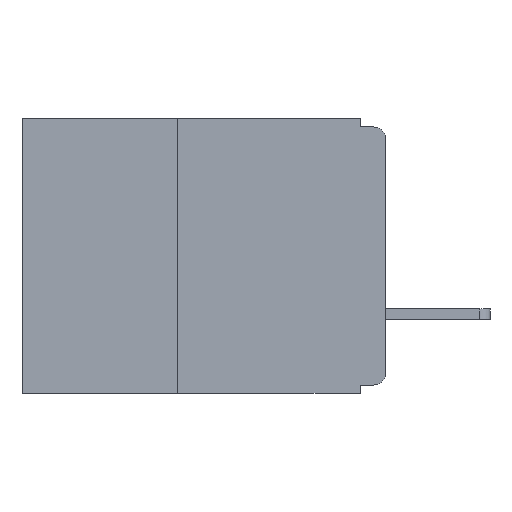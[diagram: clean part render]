
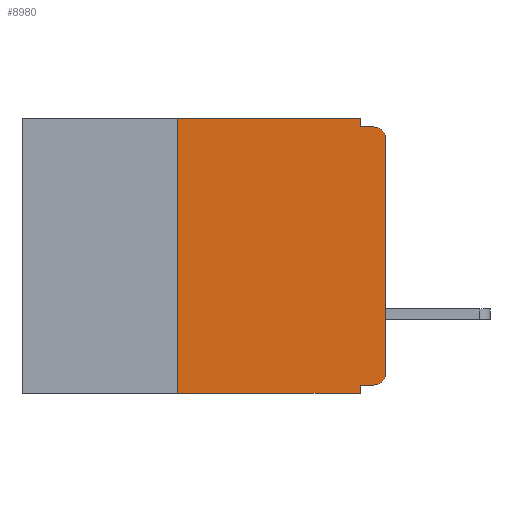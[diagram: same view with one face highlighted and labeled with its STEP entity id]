
A CAD part, left-side view. The second image highlights one B-rep face of the part: STEP entity #8980.
In plain terms, the highlighted planar face has unit normal (-1, 0, 0).
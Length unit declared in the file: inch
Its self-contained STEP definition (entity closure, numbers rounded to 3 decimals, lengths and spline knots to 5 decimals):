
#140 = CARTESIAN_POINT ( 'NONE',  ( 0., 0.031, -0.01 ) ) ;
#210 = AXIS2_PLACEMENT_3D ( 'NONE', #26010, #25913, #25876 ) ;
#274 = EDGE_CURVE ( 'NONE', #29803, #27475, #3256, .T. ) ;
#433 = ORIENTED_EDGE ( 'NONE', *, *, #26208, .T. ) ;
#924 = CARTESIAN_POINT ( 'NONE',  ( 0., 0.031, -0.33 ) ) ;
#1409 = VERTEX_POINT ( 'NONE', #28042 ) ;
#1490 = VECTOR ( 'NONE', #11071, 39.37008 ) ;
#3256 = LINE ( 'NONE', #18717, #8362 ) ;
#3645 = DIRECTION ( 'NONE',  ( 0., 0., 1. ) ) ;
#4241 = VECTOR ( 'NONE', #13066, 39.37008 ) ;
#4512 = LINE ( 'NONE', #16980, #16951 ) ;
#4658 = EDGE_CURVE ( 'NONE', #27873, #8387, #24845, .T. ) ;
#5413 = VERTEX_POINT ( 'NONE', #924 ) ;
#5503 = EDGE_LOOP ( 'NONE', ( #16473, #433, #24006, #29252, #25175, #14495, #21458, #30095, #6450, #28640 ) ) ;
#5930 = CARTESIAN_POINT ( 'NONE',  ( 0., 0.437, -0.33 ) ) ;
#6450 = ORIENTED_EDGE ( 'NONE', *, *, #13812, .F. ) ;
#6608 = CARTESIAN_POINT ( 'NONE',  ( 0., 0.015, -0.01 ) ) ;
#8142 = CARTESIAN_POINT ( 'NONE',  ( 0., 0.015, -0.025 ) ) ;
#8357 = VECTOR ( 'NONE', #3645, 39.37008 ) ;
#8362 = VECTOR ( 'NONE', #19721, 39.37008 ) ;
#8387 = VERTEX_POINT ( 'NONE', #30942 ) ;
#8980 = ADVANCED_FACE ( 'NONE', ( #16807 ), #26097, .F. ) ;
#9494 = CARTESIAN_POINT ( 'NONE',  ( 0., 0.015, -0.305 ) ) ;
#9584 = VECTOR ( 'NONE', #22092, 39.37008 ) ;
#9661 = CARTESIAN_POINT ( 'NONE',  ( 0., 0.031, -0.32 ) ) ;
#10629 = DIRECTION ( 'NONE',  ( 0., 0., -1. ) ) ;
#10862 = LINE ( 'NONE', #30079, #4241 ) ;
#11071 = DIRECTION ( 'NONE',  ( 0., 0., -1. ) ) ;
#11941 = DIRECTION ( 'NONE',  ( 0., 0., -1. ) ) ;
#13066 = DIRECTION ( 'NONE',  ( 0., -1., 0. ) ) ;
#13812 = EDGE_CURVE ( 'NONE', #22123, #22270, #4512, .T. ) ;
#13885 = EDGE_CURVE ( 'NONE', #16780, #29803, #15384, .T. ) ;
#14495 = ORIENTED_EDGE ( 'NONE', *, *, #27711, .F. ) ;
#15384 = LINE ( 'NONE', #26950, #9584 ) ;
#15468 = LINE ( 'NONE', #15939, #1490 ) ;
#15740 = CIRCLE ( 'NONE', #26552, 0.015 ) ;
#15939 = CARTESIAN_POINT ( 'NONE',  ( 0., 0.031, -0.33 ) ) ;
#16473 = ORIENTED_EDGE ( 'NONE', *, *, #4658, .T. ) ;
#16761 = VERTEX_POINT ( 'NONE', #6608 ) ;
#16780 = VERTEX_POINT ( 'NONE', #23722 ) ;
#16807 = FACE_OUTER_BOUND ( 'NONE', #5503, .T. ) ;
#16812 = CARTESIAN_POINT ( 'NONE',  ( 0., 0., -0.305 ) ) ;
#16951 = VECTOR ( 'NONE', #19457, 39.37008 ) ;
#16980 = CARTESIAN_POINT ( 'NONE',  ( 0., 0., -0.32 ) ) ;
#17456 = VECTOR ( 'NONE', #18286, 39.37008 ) ;
#18286 = DIRECTION ( 'NONE',  ( 0., -1., 0. ) ) ;
#18717 = CARTESIAN_POINT ( 'NONE',  ( 0., 0.031, 0. ) ) ;
#18892 = CARTESIAN_POINT ( 'NONE',  ( 0., 0.015, -0.32 ) ) ;
#19457 = DIRECTION ( 'NONE',  ( 0., 1., 0. ) ) ;
#19721 = DIRECTION ( 'NONE',  ( 0., 0., -1. ) ) ;
#20587 = CARTESIAN_POINT ( 'NONE',  ( 0., 0.031, 0. ) ) ;
#20899 = CARTESIAN_POINT ( 'NONE',  ( 0., 0.25, -0.33 ) ) ;
#21458 = ORIENTED_EDGE ( 'NONE', *, *, #25149, .T. ) ;
#22092 = DIRECTION ( 'NONE',  ( 0., -1., 0. ) ) ;
#22123 = VERTEX_POINT ( 'NONE', #18892 ) ;
#22270 = VERTEX_POINT ( 'NONE', #9661 ) ;
#23187 = CARTESIAN_POINT ( 'NONE',  ( 0., 0., 0. ) ) ;
#23360 = DIRECTION ( 'NONE',  ( 0., 0., 1. ) ) ;
#23722 = CARTESIAN_POINT ( 'NONE',  ( 0., 0.25, 0. ) ) ;
#24006 = ORIENTED_EDGE ( 'NONE', *, *, #25105, .F. ) ;
#24845 = LINE ( 'NONE', #23187, #30454 ) ;
#25105 = EDGE_CURVE ( 'NONE', #27475, #16761, #10862, .T. ) ;
#25149 = EDGE_CURVE ( 'NONE', #1409, #5413, #28792, .T. ) ;
#25175 = ORIENTED_EDGE ( 'NONE', *, *, #13885, .F. ) ;
#25314 = DIRECTION ( 'NONE',  ( -1., 0., 0. ) ) ;
#25789 = EDGE_CURVE ( 'NONE', #22270, #5413, #15468, .T. ) ;
#25876 = DIRECTION ( 'NONE',  ( 0., 0., -1. ) ) ;
#25913 = DIRECTION ( 'NONE',  ( 1., 0., 0. ) ) ;
#26010 = CARTESIAN_POINT ( 'NONE',  ( 0., 0.437, 0. ) ) ;
#26097 = PLANE ( 'NONE',  #210 ) ;
#26208 = EDGE_CURVE ( 'NONE', #8387, #16761, #27601, .T. ) ;
#26552 = AXIS2_PLACEMENT_3D ( 'NONE', #9494, #26610, #11941 ) ;
#26610 = DIRECTION ( 'NONE',  ( -1., 0., 0. ) ) ;
#26950 = CARTESIAN_POINT ( 'NONE',  ( 0., 0.437, 0. ) ) ;
#27314 = EDGE_CURVE ( 'NONE', #22123, #27873, #15740, .T. ) ;
#27323 = AXIS2_PLACEMENT_3D ( 'NONE', #8142, #25314, #10629 ) ;
#27475 = VERTEX_POINT ( 'NONE', #140 ) ;
#27601 = CIRCLE ( 'NONE', #27323, 0.015 ) ;
#27711 = EDGE_CURVE ( 'NONE', #1409, #16780, #27867, .T. ) ;
#27867 = LINE ( 'NONE', #20899, #8357 ) ;
#27873 = VERTEX_POINT ( 'NONE', #16812 ) ;
#28042 = CARTESIAN_POINT ( 'NONE',  ( 0., 0.25, -0.33 ) ) ;
#28640 = ORIENTED_EDGE ( 'NONE', *, *, #27314, .T. ) ;
#28792 = LINE ( 'NONE', #5930, #17456 ) ;
#29252 = ORIENTED_EDGE ( 'NONE', *, *, #274, .F. ) ;
#29803 = VERTEX_POINT ( 'NONE', #20587 ) ;
#30079 = CARTESIAN_POINT ( 'NONE',  ( 0., 0., -0.01 ) ) ;
#30095 = ORIENTED_EDGE ( 'NONE', *, *, #25789, .F. ) ;
#30454 = VECTOR ( 'NONE', #23360, 39.37008 ) ;
#30942 = CARTESIAN_POINT ( 'NONE',  ( 0., 0., -0.025 ) ) ;
